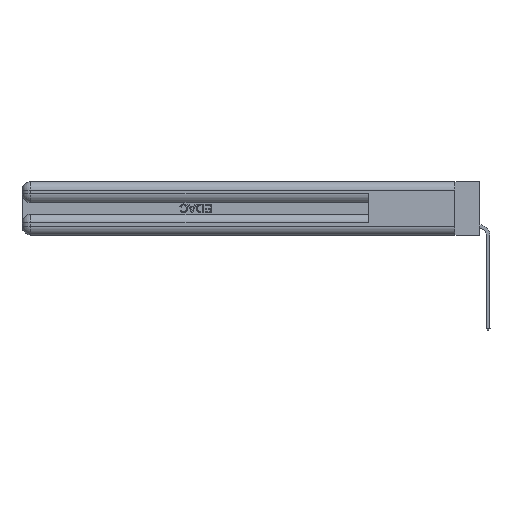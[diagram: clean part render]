
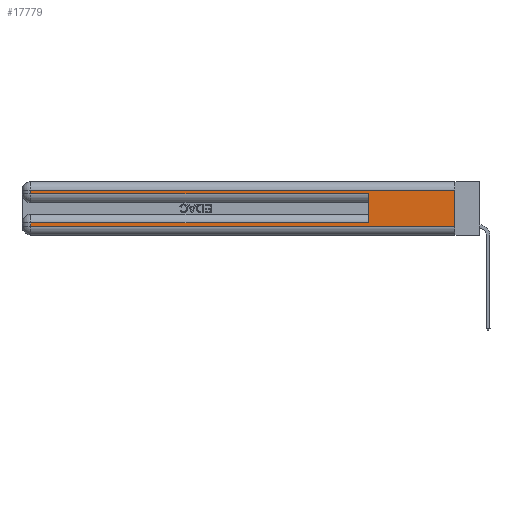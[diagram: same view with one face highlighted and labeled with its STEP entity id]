
A CAD part, left-side view. The second image highlights one B-rep face of the part: STEP entity #17779.
In plain terms, the highlighted planar face has unit normal (-1, 0, 0).
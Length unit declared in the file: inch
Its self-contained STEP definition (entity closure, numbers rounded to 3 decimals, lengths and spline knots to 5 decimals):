
#771 = CARTESIAN_POINT ( 'NONE',  ( 0., 0.6, 0.285 ) ) ;
#1505 = LINE ( 'NONE', #28595, #19081 ) ;
#1653 = VECTOR ( 'NONE', #31432, 39.37008 ) ;
#2577 = CARTESIAN_POINT ( 'NONE',  ( 0., 0., 0.31 ) ) ;
#3628 = VECTOR ( 'NONE', #28021, 39.37008 ) ;
#4397 = EDGE_CURVE ( 'NONE', #4621, #11638, #25691, .T. ) ;
#4487 = ORIENTED_EDGE ( 'NONE', *, *, #16610, .T. ) ;
#4490 = CARTESIAN_POINT ( 'NONE',  ( 0., 0., 0.06 ) ) ;
#4621 = VERTEX_POINT ( 'NONE', #31158 ) ;
#4979 = ORIENTED_EDGE ( 'NONE', *, *, #5299, .F. ) ;
#5299 = EDGE_CURVE ( 'NONE', #10932, #23718, #9727, .T. ) ;
#5429 = CARTESIAN_POINT ( 'NONE',  ( 0., 0.6, 0.085 ) ) ;
#6317 = AXIS2_PLACEMENT_3D ( 'NONE', #10613, #18364, #18205 ) ;
#6511 = EDGE_CURVE ( 'NONE', #16352, #4621, #18511, .T. ) ;
#6513 = DIRECTION ( 'NONE',  ( 0., 0., -1. ) ) ;
#7385 = CARTESIAN_POINT ( 'NONE',  ( 0., 0., 0.285 ) ) ;
#8239 = CARTESIAN_POINT ( 'NONE',  ( 0., 2.94, 0.37 ) ) ;
#8508 = PLANE ( 'NONE',  #6317 ) ;
#8595 = EDGE_CURVE ( 'NONE', #10932, #14586, #1505, .T. ) ;
#8666 = CARTESIAN_POINT ( 'NONE',  ( 0., 0., 0.06 ) ) ;
#8746 = DIRECTION ( 'NONE',  ( 0., 1., 0. ) ) ;
#9727 = LINE ( 'NONE', #21843, #31578 ) ;
#10158 = VECTOR ( 'NONE', #20141, 39.37008 ) ;
#10613 = CARTESIAN_POINT ( 'NONE',  ( 0., 0., 0.37 ) ) ;
#10932 = VERTEX_POINT ( 'NONE', #5429 ) ;
#11149 = DIRECTION ( 'NONE',  ( 0., 0., -1. ) ) ;
#11638 = VERTEX_POINT ( 'NONE', #19216 ) ;
#11659 = VECTOR ( 'NONE', #27813, 39.37008 ) ;
#13202 = ORIENTED_EDGE ( 'NONE', *, *, #6511, .T. ) ;
#14586 = VERTEX_POINT ( 'NONE', #28743 ) ;
#14943 = CARTESIAN_POINT ( 'NONE',  ( 0., 2.94, 0.06 ) ) ;
#15302 = ORIENTED_EDGE ( 'NONE', *, *, #29695, .F. ) ;
#16268 = VECTOR ( 'NONE', #6513, 39.37008 ) ;
#16352 = VERTEX_POINT ( 'NONE', #2577 ) ;
#16360 = ORIENTED_EDGE ( 'NONE', *, *, #4397, .T. ) ;
#16610 = EDGE_CURVE ( 'NONE', #24510, #19863, #30954, .T. ) ;
#17779 = ADVANCED_FACE ( 'NONE', ( #23375 ), #8508, .F. ) ;
#17805 = ORIENTED_EDGE ( 'NONE', *, *, #30448, .T. ) ;
#17970 = LINE ( 'NONE', #20250, #11659 ) ;
#18205 = DIRECTION ( 'NONE',  ( 0., 0., -1. ) ) ;
#18364 = DIRECTION ( 'NONE',  ( 1., 0., 0. ) ) ;
#18511 = LINE ( 'NONE', #23197, #3628 ) ;
#19081 = VECTOR ( 'NONE', #8746, 39.37008 ) ;
#19216 = CARTESIAN_POINT ( 'NONE',  ( 0., 2.94, 0.285 ) ) ;
#19863 = VERTEX_POINT ( 'NONE', #4490 ) ;
#20141 = DIRECTION ( 'NONE',  ( 0., -1., 0. ) ) ;
#20250 = CARTESIAN_POINT ( 'NONE',  ( 0., 0., 0.37 ) ) ;
#21843 = CARTESIAN_POINT ( 'NONE',  ( 0., 0.6, 0.145 ) ) ;
#21980 = EDGE_CURVE ( 'NONE', #14586, #24510, #31066, .T. ) ;
#23197 = CARTESIAN_POINT ( 'NONE',  ( 0., 0., 0.31 ) ) ;
#23375 = FACE_OUTER_BOUND ( 'NONE', #29616, .T. ) ;
#23718 = VERTEX_POINT ( 'NONE', #771 ) ;
#23999 = ORIENTED_EDGE ( 'NONE', *, *, #8595, .T. ) ;
#24510 = VERTEX_POINT ( 'NONE', #14943 ) ;
#25691 = LINE ( 'NONE', #8239, #27212 ) ;
#25912 = ORIENTED_EDGE ( 'NONE', *, *, #21980, .T. ) ;
#26934 = LINE ( 'NONE', #7385, #10158 ) ;
#27212 = VECTOR ( 'NONE', #11149, 39.37008 ) ;
#27813 = DIRECTION ( 'NONE',  ( 0., 0., -1. ) ) ;
#28021 = DIRECTION ( 'NONE',  ( 0., 1., 0. ) ) ;
#28595 = CARTESIAN_POINT ( 'NONE',  ( 0., 0., 0.085 ) ) ;
#28628 = CARTESIAN_POINT ( 'NONE',  ( 0., 2.94, 0.37 ) ) ;
#28743 = CARTESIAN_POINT ( 'NONE',  ( 0., 2.94, 0.085 ) ) ;
#29578 = DIRECTION ( 'NONE',  ( 0., 0., 1. ) ) ;
#29616 = EDGE_LOOP ( 'NONE', ( #15302, #13202, #16360, #17805, #4979, #23999, #25912, #4487 ) ) ;
#29695 = EDGE_CURVE ( 'NONE', #16352, #19863, #17970, .T. ) ;
#30448 = EDGE_CURVE ( 'NONE', #11638, #23718, #26934, .T. ) ;
#30954 = LINE ( 'NONE', #8666, #1653 ) ;
#31066 = LINE ( 'NONE', #28628, #16268 ) ;
#31158 = CARTESIAN_POINT ( 'NONE',  ( 0., 2.94, 0.31 ) ) ;
#31432 = DIRECTION ( 'NONE',  ( 0., -1., 0. ) ) ;
#31578 = VECTOR ( 'NONE', #29578, 39.37008 ) ;
